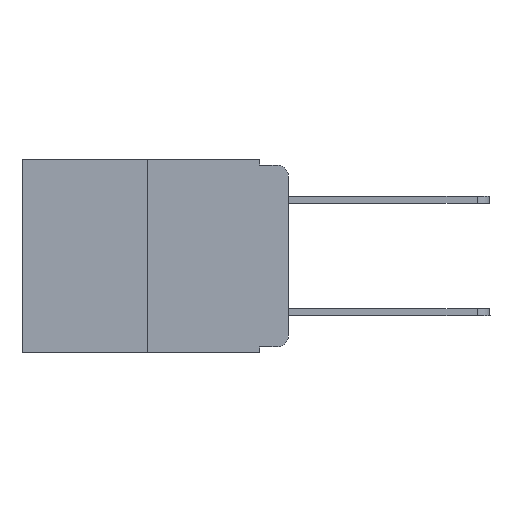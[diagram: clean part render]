
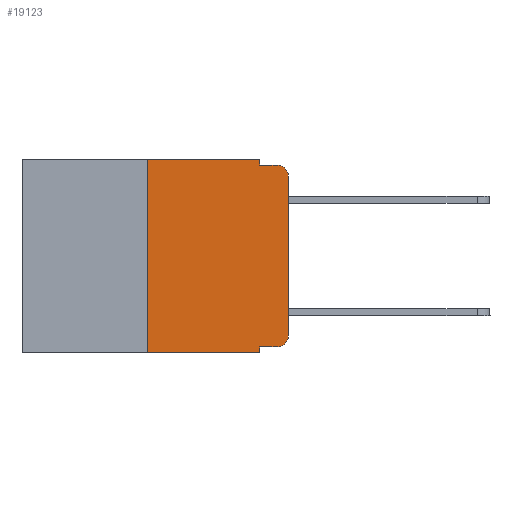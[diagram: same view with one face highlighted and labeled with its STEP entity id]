
A CAD part, left-side view. The second image highlights one B-rep face of the part: STEP entity #19123.
In plain terms, the highlighted planar face has unit normal (-1, 0, 0).
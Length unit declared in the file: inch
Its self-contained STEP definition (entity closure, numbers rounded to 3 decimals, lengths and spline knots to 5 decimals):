
#229 = CARTESIAN_POINT ( 'NONE',  ( 0., 0.473, -0.343 ) ) ;
#426 = ORIENTED_EDGE ( 'NONE', *, *, #14315, .T. ) ;
#520 = VECTOR ( 'NONE', #17606, 39.37008 ) ;
#540 = VECTOR ( 'NONE', #6494, 39.37008 ) ;
#699 = CARTESIAN_POINT ( 'NONE',  ( 0., 0.25, -0.343 ) ) ;
#910 = DIRECTION ( 'NONE',  ( 0., 0., -1. ) ) ;
#1281 = EDGE_CURVE ( 'NONE', #11522, #11285, #17961, .T. ) ;
#1462 = DIRECTION ( 'NONE',  ( -1., 0., 0. ) ) ;
#1465 = CARTESIAN_POINT ( 'NONE',  ( 0., 0.473, 0. ) ) ;
#1490 = VERTEX_POINT ( 'NONE', #19382 ) ;
#1572 = CARTESIAN_POINT ( 'NONE',  ( 0., 0.051, -0.333 ) ) ;
#2050 = LINE ( 'NONE', #20643, #540 ) ;
#2727 = ORIENTED_EDGE ( 'NONE', *, *, #14157, .F. ) ;
#3042 = CARTESIAN_POINT ( 'NONE',  ( 0., 0.051, 0. ) ) ;
#3053 = VERTEX_POINT ( 'NONE', #4117 ) ;
#3411 = EDGE_CURVE ( 'NONE', #17582, #8744, #16087, .T. ) ;
#3485 = AXIS2_PLACEMENT_3D ( 'NONE', #1465, #12846, #7980 ) ;
#4117 = CARTESIAN_POINT ( 'NONE',  ( 0., 0., -0.03 ) ) ;
#4365 = CARTESIAN_POINT ( 'NONE',  ( 0., 0.051, 0. ) ) ;
#4579 = DIRECTION ( 'NONE',  ( 0., 0., 1. ) ) ;
#4582 = VECTOR ( 'NONE', #4579, 39.37008 ) ;
#4983 = LINE ( 'NONE', #229, #11269 ) ;
#5589 = DIRECTION ( 'NONE',  ( -1., 0., 0. ) ) ;
#5903 = VERTEX_POINT ( 'NONE', #14888 ) ;
#6192 = CARTESIAN_POINT ( 'NONE',  ( 0., 0.25, 0. ) ) ;
#6236 = PLANE ( 'NONE',  #3485 ) ;
#6339 = CARTESIAN_POINT ( 'NONE',  ( 0., 0.473, 0. ) ) ;
#6494 = DIRECTION ( 'NONE',  ( 0., -1., 0. ) ) ;
#6668 = VECTOR ( 'NONE', #14856, 39.37008 ) ;
#7162 = CARTESIAN_POINT ( 'NONE',  ( 0., 0., -0.313 ) ) ;
#7383 = VECTOR ( 'NONE', #10819, 39.37008 ) ;
#7526 = VECTOR ( 'NONE', #19849, 39.37008 ) ;
#7980 = DIRECTION ( 'NONE',  ( 0., 0., -1. ) ) ;
#8277 = ORIENTED_EDGE ( 'NONE', *, *, #13506, .T. ) ;
#8420 = ORIENTED_EDGE ( 'NONE', *, *, #16868, .T. ) ;
#8744 = VERTEX_POINT ( 'NONE', #10065 ) ;
#8881 = CIRCLE ( 'NONE', #20750, 0.02 ) ;
#9597 = DIRECTION ( 'NONE',  ( 0., 0., -1. ) ) ;
#10065 = CARTESIAN_POINT ( 'NONE',  ( 0., 0.051, -0.343 ) ) ;
#10138 = VERTEX_POINT ( 'NONE', #7162 ) ;
#10171 = DIRECTION ( 'NONE',  ( 0., -1., 0. ) ) ;
#10359 = ORIENTED_EDGE ( 'NONE', *, *, #14308, .F. ) ;
#10367 = EDGE_CURVE ( 'NONE', #11953, #20351, #11678, .T. ) ;
#10769 = DIRECTION ( 'NONE',  ( 0., -1., 0. ) ) ;
#10819 = DIRECTION ( 'NONE',  ( 0., 0., -1. ) ) ;
#11269 = VECTOR ( 'NONE', #10171, 39.37008 ) ;
#11285 = VERTEX_POINT ( 'NONE', #13774 ) ;
#11480 = CARTESIAN_POINT ( 'NONE',  ( 0., 0.25, 0. ) ) ;
#11522 = VERTEX_POINT ( 'NONE', #3042 ) ;
#11545 = ORIENTED_EDGE ( 'NONE', *, *, #1281, .F. ) ;
#11678 = LINE ( 'NONE', #11480, #6668 ) ;
#11842 = EDGE_LOOP ( 'NONE', ( #426, #8420, #2727, #11545, #10359, #16538, #18433, #14829, #8277, #19582 ) ) ;
#11953 = VERTEX_POINT ( 'NONE', #699 ) ;
#11980 = CARTESIAN_POINT ( 'NONE',  ( 0., 0.02, -0.313 ) ) ;
#12643 = LINE ( 'NONE', #6339, #520 ) ;
#12846 = DIRECTION ( 'NONE',  ( 1., 0., 0. ) ) ;
#12905 = LINE ( 'NONE', #15693, #17439 ) ;
#13263 = CARTESIAN_POINT ( 'NONE',  ( 0., 0.051, 0. ) ) ;
#13506 = EDGE_CURVE ( 'NONE', #17582, #5903, #2050, .T. ) ;
#13774 = CARTESIAN_POINT ( 'NONE',  ( 0., 0.051, -0.01 ) ) ;
#14157 = EDGE_CURVE ( 'NONE', #11285, #1490, #12905, .T. ) ;
#14195 = FACE_OUTER_BOUND ( 'NONE', #11842, .T. ) ;
#14308 = EDGE_CURVE ( 'NONE', #20351, #11522, #12643, .T. ) ;
#14315 = EDGE_CURVE ( 'NONE', #10138, #3053, #15387, .T. ) ;
#14829 = ORIENTED_EDGE ( 'NONE', *, *, #3411, .F. ) ;
#14856 = DIRECTION ( 'NONE',  ( 0., 0., 1. ) ) ;
#14888 = CARTESIAN_POINT ( 'NONE',  ( 0., 0.02, -0.333 ) ) ;
#15387 = LINE ( 'NONE', #16123, #4582 ) ;
#15444 = AXIS2_PLACEMENT_3D ( 'NONE', #20781, #1462, #9597 ) ;
#15693 = CARTESIAN_POINT ( 'NONE',  ( 0., 0.051, -0.01 ) ) ;
#15858 = EDGE_CURVE ( 'NONE', #11953, #8744, #4983, .T. ) ;
#16087 = LINE ( 'NONE', #13263, #7526 ) ;
#16123 = CARTESIAN_POINT ( 'NONE',  ( 0., 0., 0. ) ) ;
#16538 = ORIENTED_EDGE ( 'NONE', *, *, #10367, .F. ) ;
#16868 = EDGE_CURVE ( 'NONE', #3053, #1490, #18795, .T. ) ;
#17439 = VECTOR ( 'NONE', #10769, 39.37008 ) ;
#17582 = VERTEX_POINT ( 'NONE', #1572 ) ;
#17606 = DIRECTION ( 'NONE',  ( 0., -1., 0. ) ) ;
#17961 = LINE ( 'NONE', #4365, #7383 ) ;
#18433 = ORIENTED_EDGE ( 'NONE', *, *, #15858, .T. ) ;
#18795 = CIRCLE ( 'NONE', #15444, 0.02 ) ;
#19123 = ADVANCED_FACE ( 'NONE', ( #14195 ), #6236, .F. ) ;
#19382 = CARTESIAN_POINT ( 'NONE',  ( 0., 0.02, -0.01 ) ) ;
#19439 = EDGE_CURVE ( 'NONE', #5903, #10138, #8881, .T. ) ;
#19582 = ORIENTED_EDGE ( 'NONE', *, *, #19439, .T. ) ;
#19849 = DIRECTION ( 'NONE',  ( 0., 0., -1. ) ) ;
#20351 = VERTEX_POINT ( 'NONE', #6192 ) ;
#20643 = CARTESIAN_POINT ( 'NONE',  ( 0., 0.051, -0.333 ) ) ;
#20750 = AXIS2_PLACEMENT_3D ( 'NONE', #11980, #5589, #910 ) ;
#20781 = CARTESIAN_POINT ( 'NONE',  ( 0., 0.02, -0.03 ) ) ;
